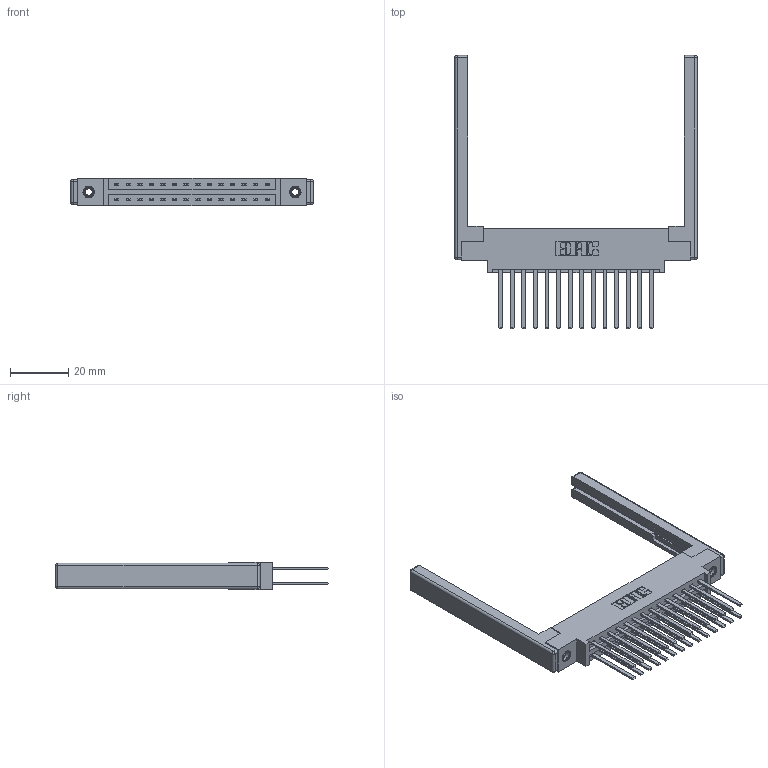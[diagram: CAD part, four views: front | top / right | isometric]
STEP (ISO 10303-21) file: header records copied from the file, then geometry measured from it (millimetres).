
FILE_DESCRIPTION (( 'STEP AP203' ), '1' );
FILE_NAME ('337-028-544-868.STEP', '2019-10-10T22:56:21', ( '' ), ( '' ), 'SwSTEP 2.0', 'SolidWorks 2016', '' );
FILE_SCHEMA (( 'CONFIG_CONTROL_DESIGN' ));
Length unit declared in the file: inch
Products named in the file (5): 307-220-068; 337-028-544-868; 345-250-001_345-250-001-102; 345-292-001_345-293-144; 337 Part_0.170 Offset - 0.156 Dia-TI
Assembly tree (33 placements, depth 2):
  337-028-544-868
    337 Part_0.170 Offset - 0.156 Dia-TI
    345-292-001_345-293-144  x28
    345-250-001_345-250-001-102  x2
    307-220-068  x2
Bounding box: 82.91 x 93.35 x 9.4 mm (x, y, z)
Volume: 13024.3 mm3; surface area: 14919.5 mm2
Topology: 33 solids, 33 shells, 1616 faces, 4717 edges, 3086 vertices
Faces by surface type: plane 1114, cylinder 478, cone 12, sphere 8, torus 4
Entity records: 17184 total; most frequent: CARTESIAN_POINT 2883, ORIENTED_EDGE 2808, DIRECTION 2570, EDGE_CURVE 1404, LINE 1230, VECTOR 1230, VERTEX_POINT 926, AXIS2_PLACEMENT_3D 670
